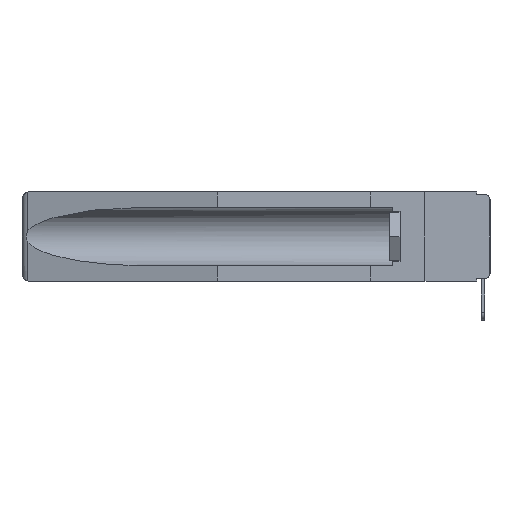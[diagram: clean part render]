
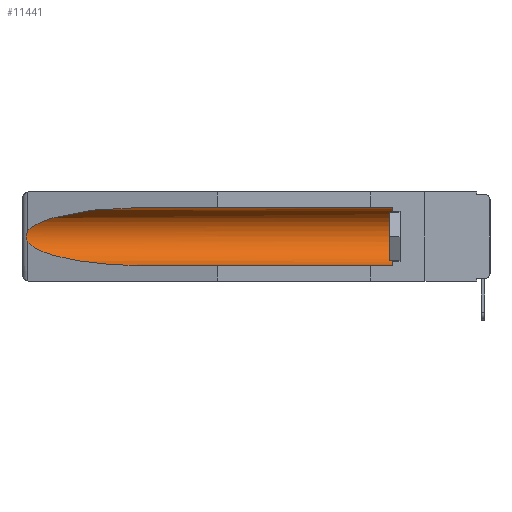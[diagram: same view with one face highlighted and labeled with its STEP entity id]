
A CAD part, left-side view. The second image highlights one B-rep face of the part: STEP entity #11441.
In plain terms, the highlighted cylindrical face has radius 2.857 mm (diameter 5.715 mm), a partial arc.
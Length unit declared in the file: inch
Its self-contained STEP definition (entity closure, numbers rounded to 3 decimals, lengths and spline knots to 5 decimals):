
#130 = CARTESIAN_POINT ( 'NONE',  ( 0.26537, 1.52718, -0.14972 ) ) ;
#825 = VERTEX_POINT ( 'NONE', #2193 ) ;
#1103 = CARTESIAN_POINT ( 'NONE',  ( 0.155, 1.07973, -0.059 ) ) ;
#1244 = CARTESIAN_POINT ( 'NONE',  ( 0.155, -0.30754, -0.059 ) ) ;
#1871 = CARTESIAN_POINT ( 'NONE',  ( 0.26597, 1.5296, -0.19026 ) ) ;
#2193 = CARTESIAN_POINT ( 'NONE',  ( 0.155, 0.126, -0.059 ) ) ;
#2448 = VERTEX_POINT ( 'NONE', #21202 ) ;
#2881 = CARTESIAN_POINT ( 'NONE',  ( 0.26537, 1.52718, -0.19328 ) ) ;
#3065 = DIRECTION ( 'NONE',  ( 0., 0., 1. ) ) ;
#3076 = VERTEX_POINT ( 'NONE', #17681 ) ;
#3362 = EDGE_CURVE ( 'NONE', #3076, #825, #11911, .T. ) ;
#3665 = CARTESIAN_POINT ( 'NONE',  ( 0.2673, 1.5327, -0.16383 ) ) ;
#4641 = CARTESIAN_POINT ( 'NONE',  ( 0.21114, 1.30732, -0.059 ) ) ;
#4773 = CARTESIAN_POINT ( 'NONE',  ( 0.26537, 1.52718, -0.14972 ) ) ;
#5436 = EDGE_CURVE ( 'NONE', #3076, #2448, #7755, .T. ) ;
#6191 = ORIENTED_EDGE ( 'NONE', *, *, #7201, .T. ) ;
#6434 = CARTESIAN_POINT ( 'NONE',  ( 0.155, 1.07973, -0.284 ) ) ;
#6730 = EDGE_CURVE ( 'NONE', #825, #15956, #7149, .T. ) ;
#7149 = LINE ( 'NONE', #1244, #14771 ) ;
#7201 = EDGE_CURVE ( 'NONE', #12204, #2448, #19961, .T. ) ;
#7352 = CARTESIAN_POINT ( 'NONE',  ( 0.2675, 1.53308, -0.17534 ) ) ;
#7628 = ORIENTED_EDGE ( 'NONE', *, *, #11083, .T. ) ;
#7755 = LINE ( 'NONE', #15205, #13214 ) ;
#7998 = CARTESIAN_POINT ( 'NONE',  ( 0.21114, 1.30732, -0.284 ) ) ;
#8077 = CARTESIAN_POINT ( 'NONE',  ( 0.25451, 1.48313, -0.24835 ) ) ;
#8114 = CARTESIAN_POINT ( 'NONE',  ( 0.26537, 1.52718, -0.14972 ) ) ;
#8272 = FACE_OUTER_BOUND ( 'NONE', #18921, .T. ) ;
#8869 = VERTEX_POINT ( 'NONE', #4773 ) ;
#9046 = ORIENTED_EDGE ( 'NONE', *, *, #3362, .T. ) ;
#9993 = CARTESIAN_POINT ( 'NONE',  ( 0.25451, 1.48313, -0.09465 ) ) ;
#10605 = CARTESIAN_POINT ( 'NONE',  ( 0.26537, 1.52718, -0.19328 ) ) ;
#10683 = CARTESIAN_POINT ( 'NONE',  ( 0.2673, 1.53269, -0.17917 ) ) ;
#11083 = EDGE_CURVE ( 'NONE', #8869, #12204, #19263, .T. ) ;
#11441 = ADVANCED_FACE ( 'NONE', ( #8272 ), #15097, .F. ) ;
#11911 = CIRCLE ( 'NONE', #14123, 0.1125 ) ;
#11982 = DIRECTION ( 'NONE',  ( 0., 1., 0. ) ) ;
#12204 = VERTEX_POINT ( 'NONE', #2881 ) ;
#12299 = CARTESIAN_POINT ( 'NONE',  ( 0.2675, 1.53308, -0.16763 ) ) ;
#13214 = VECTOR ( 'NONE', #21945, 39.37008 ) ;
#13266 = ORIENTED_EDGE ( 'NONE', *, *, #17063, .T. ) ;
#13271 = CARTESIAN_POINT ( 'NONE',  ( 0.26537, 1.52718, -0.19328 ) ) ;
#13413 = CARTESIAN_POINT ( 'NONE',  ( 0.155, 1.07973, -0.059 ) ) ;
#13985 =( BOUNDED_CURVE ( )  B_SPLINE_CURVE ( 3, ( #1103, #4641, #9993, #8114 ),
 .UNSPECIFIED., .F., .T. ) 
 B_SPLINE_CURVE_WITH_KNOTS ( ( 4, 4 ),
 ( 4.71239, 6.08839 ),
 .UNSPECIFIED. ) 
 CURVE ( )  GEOMETRIC_REPRESENTATION_ITEM ( )  RATIONAL_B_SPLINE_CURVE ( ( 1., 0.848, 0.848, 1. ) ) 
 REPRESENTATION_ITEM ( '' )  );
#14123 = AXIS2_PLACEMENT_3D ( 'NONE', #16965, #15072, #3065 ) ;
#14150 = CARTESIAN_POINT ( 'NONE',  ( 0.26655, 1.53094, -0.18657 ) ) ;
#14218 = CARTESIAN_POINT ( 'NONE',  ( 0.26654, 1.53092, -0.15636 ) ) ;
#14771 = VECTOR ( 'NONE', #18521, 39.37008 ) ;
#15072 = DIRECTION ( 'NONE',  ( 0., -1., 0. ) ) ;
#15097 = CYLINDRICAL_SURFACE ( 'NONE', #21223, 0.1125 ) ;
#15205 = CARTESIAN_POINT ( 'NONE',  ( 0.155, -0.30754, -0.284 ) ) ;
#15508 = DIRECTION ( 'NONE',  ( 0., 0., 1. ) ) ;
#15956 = VERTEX_POINT ( 'NONE', #13413 ) ;
#15968 = CARTESIAN_POINT ( 'NONE',  ( 0.26597, 1.52961, -0.15275 ) ) ;
#16965 = CARTESIAN_POINT ( 'NONE',  ( 0.155, 0.126, -0.1715 ) ) ;
#17063 = EDGE_CURVE ( 'NONE', #15956, #8869, #13985, .T. ) ;
#17308 = ORIENTED_EDGE ( 'NONE', *, *, #6730, .T. ) ;
#17681 = CARTESIAN_POINT ( 'NONE',  ( 0.155, 0.126, -0.284 ) ) ;
#18521 = DIRECTION ( 'NONE',  ( 0., 1., 0. ) ) ;
#18921 = EDGE_LOOP ( 'NONE', ( #13266, #7628, #6191, #21727, #9046, #17308 ) ) ;
#19263 = B_SPLINE_CURVE_WITH_KNOTS ( 'NONE', 3,
 ( #130, #15968, #14218, #3665, #12299, #7352, #10683, #14150, #1871, #10605 ),
 .UNSPECIFIED., .F., .F.,
 ( 4, 2, 2, 2, 4 ),
 ( 0., 0.00029, 0.00058, 0.00087, 0.00117 ),
 .UNSPECIFIED. ) ;
#19961 =( BOUNDED_CURVE ( )  B_SPLINE_CURVE ( 3, ( #13271, #8077, #7998, #6434 ),
 .UNSPECIFIED., .F., .F. ) 
 B_SPLINE_CURVE_WITH_KNOTS ( ( 4, 4 ),
 ( 0.1948, 1.5708 ),
 .UNSPECIFIED. ) 
 CURVE ( )  GEOMETRIC_REPRESENTATION_ITEM ( )  RATIONAL_B_SPLINE_CURVE ( ( 1., 0.848, 0.848, 1. ) ) 
 REPRESENTATION_ITEM ( '' )  );
#20860 = CARTESIAN_POINT ( 'NONE',  ( 0.155, -0.30754, -0.1715 ) ) ;
#21202 = CARTESIAN_POINT ( 'NONE',  ( 0.155, 1.07973, -0.284 ) ) ;
#21223 = AXIS2_PLACEMENT_3D ( 'NONE', #20860, #11982, #15508 ) ;
#21727 = ORIENTED_EDGE ( 'NONE', *, *, #5436, .F. ) ;
#21945 = DIRECTION ( 'NONE',  ( 0., 1., 0. ) ) ;
